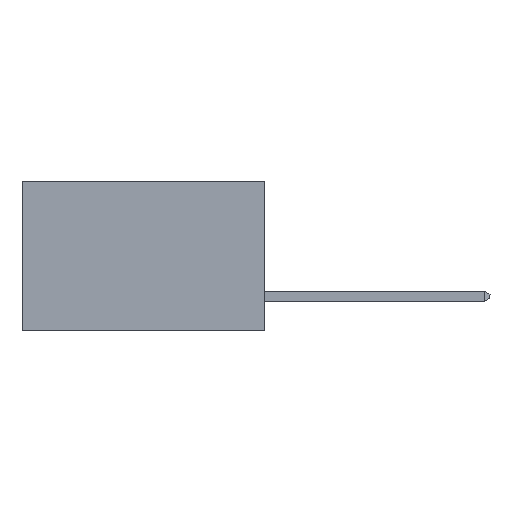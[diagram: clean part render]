
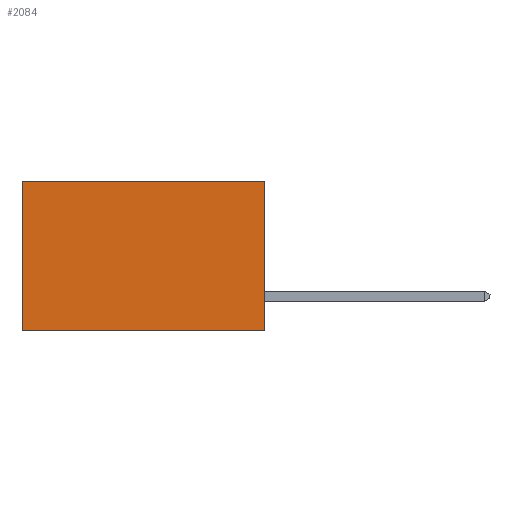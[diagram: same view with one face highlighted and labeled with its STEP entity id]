
A CAD part, left-side view. The second image highlights one B-rep face of the part: STEP entity #2084.
In plain terms, the highlighted planar face has unit normal (-1, 0, 0).
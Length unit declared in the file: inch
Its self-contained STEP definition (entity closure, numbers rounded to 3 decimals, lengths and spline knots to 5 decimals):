
#101 = CARTESIAN_POINT ( 'NONE',  ( 0.2615, 0., -0.37 ) ) ;
#246 = VECTOR ( 'NONE', #9021, 39.37008 ) ;
#355 = EDGE_CURVE ( 'NONE', #4515, #4534, #2779, .T. ) ;
#417 = CARTESIAN_POINT ( 'NONE',  ( 0.2615, 0.6, -0.37 ) ) ;
#501 = DIRECTION ( 'NONE',  ( 0., 1., 0. ) ) ;
#1242 = CARTESIAN_POINT ( 'NONE',  ( 0.2615, 0.6, -0.37 ) ) ;
#1436 = LINE ( 'NONE', #3572, #246 ) ;
#1842 = VECTOR ( 'NONE', #4668, 39.37008 ) ;
#1950 = DIRECTION ( 'NONE',  ( 1., 0., 0. ) ) ;
#2084 = ADVANCED_FACE ( 'NONE', ( #8904 ), #5435, .F. ) ;
#2779 = LINE ( 'NONE', #101, #7957 ) ;
#2928 = VERTEX_POINT ( 'NONE', #3302 ) ;
#3274 = ORIENTED_EDGE ( 'NONE', *, *, #4502, .T. ) ;
#3302 = CARTESIAN_POINT ( 'NONE',  ( 0.2615, 0.6, 0. ) ) ;
#3546 = DIRECTION ( 'NONE',  ( 0., 0., -1. ) ) ;
#3572 = CARTESIAN_POINT ( 'NONE',  ( 0.2615, 0., -0.37 ) ) ;
#3756 = VERTEX_POINT ( 'NONE', #3997 ) ;
#3997 = CARTESIAN_POINT ( 'NONE',  ( 0.2615, 0., 0. ) ) ;
#4502 = EDGE_CURVE ( 'NONE', #3756, #2928, #4712, .T. ) ;
#4515 = VERTEX_POINT ( 'NONE', #5412 ) ;
#4522 = EDGE_CURVE ( 'NONE', #2928, #4534, #7324, .T. ) ;
#4534 = VERTEX_POINT ( 'NONE', #1242 ) ;
#4668 = DIRECTION ( 'NONE',  ( 0., 0., -1. ) ) ;
#4712 = LINE ( 'NONE', #5317, #6069 ) ;
#5160 = ORIENTED_EDGE ( 'NONE', *, *, #4522, .T. ) ;
#5286 = ORIENTED_EDGE ( 'NONE', *, *, #6411, .F. ) ;
#5317 = CARTESIAN_POINT ( 'NONE',  ( 0.2615, 0., 0. ) ) ;
#5412 = CARTESIAN_POINT ( 'NONE',  ( 0.2615, 0., -0.37 ) ) ;
#5435 = PLANE ( 'NONE',  #7416 ) ;
#6069 = VECTOR ( 'NONE', #501, 39.37008 ) ;
#6169 = ORIENTED_EDGE ( 'NONE', *, *, #355, .F. ) ;
#6411 = EDGE_CURVE ( 'NONE', #3756, #4515, #1436, .T. ) ;
#7324 = LINE ( 'NONE', #417, #1842 ) ;
#7416 = AXIS2_PLACEMENT_3D ( 'NONE', #8215, #1950, #3546 ) ;
#7957 = VECTOR ( 'NONE', #8344, 39.37008 ) ;
#8215 = CARTESIAN_POINT ( 'NONE',  ( 0.2615, 0., -0.37 ) ) ;
#8344 = DIRECTION ( 'NONE',  ( 0., 1., 0. ) ) ;
#8789 = EDGE_LOOP ( 'NONE', ( #5160, #6169, #5286, #3274 ) ) ;
#8904 = FACE_OUTER_BOUND ( 'NONE', #8789, .T. ) ;
#9021 = DIRECTION ( 'NONE',  ( 0., 0., -1. ) ) ;
